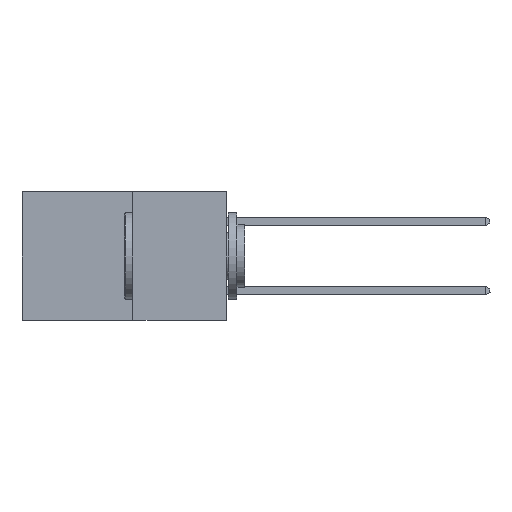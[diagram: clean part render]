
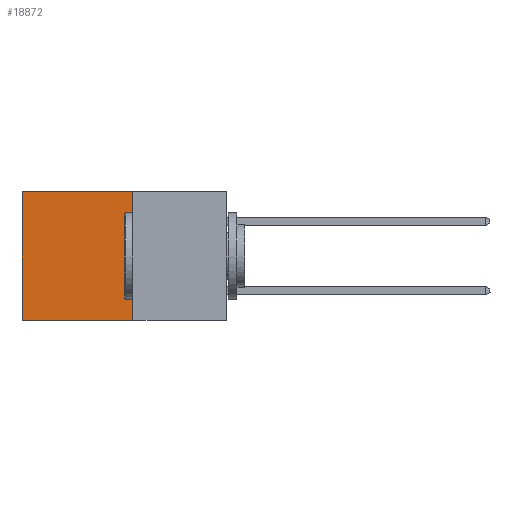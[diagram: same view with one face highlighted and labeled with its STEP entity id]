
A CAD part, left-side view. The second image highlights one B-rep face of the part: STEP entity #18872.
In plain terms, the highlighted planar face has unit normal (-1, 0, 0).
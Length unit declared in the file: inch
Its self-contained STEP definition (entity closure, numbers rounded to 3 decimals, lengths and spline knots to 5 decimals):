
#498 = VECTOR ( 'NONE', #15933, 39.37008 ) ;
#887 = VECTOR ( 'NONE', #7260, 39.37008 ) ;
#901 = EDGE_CURVE ( 'NONE', #5631, #8573, #20956, .T. ) ;
#1269 = CARTESIAN_POINT ( 'NONE',  ( 0.277, 0.27, 0. ) ) ;
#3066 = EDGE_CURVE ( 'NONE', #8573, #10112, #19065, .T. ) ;
#3336 = PLANE ( 'NONE',  #6942 ) ;
#5337 = DIRECTION ( 'NONE',  ( 0., 1., 0. ) ) ;
#5631 = VERTEX_POINT ( 'NONE', #26161 ) ;
#6942 = AXIS2_PLACEMENT_3D ( 'NONE', #8194, #24055, #10518 ) ;
#7129 = CARTESIAN_POINT ( 'NONE',  ( 0.277, 0.59, 0. ) ) ;
#7260 = DIRECTION ( 'NONE',  ( 0., 1., 0. ) ) ;
#7539 = LINE ( 'NONE', #27158, #498 ) ;
#7659 = VECTOR ( 'NONE', #22300, 39.37008 ) ;
#8182 = CARTESIAN_POINT ( 'NONE',  ( 0.277, 0.59, -0.37 ) ) ;
#8194 = CARTESIAN_POINT ( 'NONE',  ( 0.277, 0.27, -0.37 ) ) ;
#8483 = EDGE_CURVE ( 'NONE', #5631, #17349, #7539, .T. ) ;
#8573 = VERTEX_POINT ( 'NONE', #7129 ) ;
#10112 = VERTEX_POINT ( 'NONE', #8182 ) ;
#10518 = DIRECTION ( 'NONE',  ( 0., 0., -1. ) ) ;
#14458 = CARTESIAN_POINT ( 'NONE',  ( 0.277, 0.27, -0.37 ) ) ;
#15534 = FACE_OUTER_BOUND ( 'NONE', #17391, .T. ) ;
#15933 = DIRECTION ( 'NONE',  ( 0., 0., -1. ) ) ;
#17349 = VERTEX_POINT ( 'NONE', #14458 ) ;
#17391 = EDGE_LOOP ( 'NONE', ( #21453, #21139, #29443, #19185 ) ) ;
#18872 = ADVANCED_FACE ( 'NONE', ( #15534 ), #3336, .F. ) ;
#19065 = LINE ( 'NONE', #22360, #7659 ) ;
#19185 = ORIENTED_EDGE ( 'NONE', *, *, #901, .T. ) ;
#20753 = EDGE_CURVE ( 'NONE', #17349, #10112, #24576, .T. ) ;
#20887 = CARTESIAN_POINT ( 'NONE',  ( 0.277, 0.27, -0.37 ) ) ;
#20956 = LINE ( 'NONE', #1269, #25516 ) ;
#21139 = ORIENTED_EDGE ( 'NONE', *, *, #20753, .F. ) ;
#21453 = ORIENTED_EDGE ( 'NONE', *, *, #3066, .T. ) ;
#22300 = DIRECTION ( 'NONE',  ( 0., 0., -1. ) ) ;
#22360 = CARTESIAN_POINT ( 'NONE',  ( 0.277, 0.59, -0.37 ) ) ;
#24055 = DIRECTION ( 'NONE',  ( 1., 0., 0. ) ) ;
#24576 = LINE ( 'NONE', #20887, #887 ) ;
#25516 = VECTOR ( 'NONE', #5337, 39.37008 ) ;
#26161 = CARTESIAN_POINT ( 'NONE',  ( 0.277, 0.27, 0. ) ) ;
#27158 = CARTESIAN_POINT ( 'NONE',  ( 0.277, 0.27, -0.37 ) ) ;
#29443 = ORIENTED_EDGE ( 'NONE', *, *, #8483, .F. ) ;
